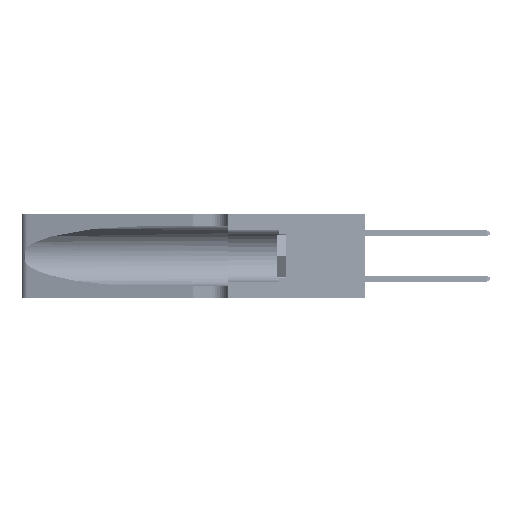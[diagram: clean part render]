
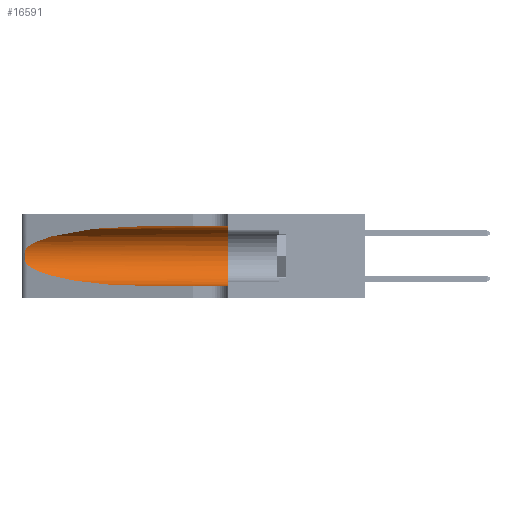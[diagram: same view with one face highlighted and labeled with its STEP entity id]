
A CAD part, left-side view. The second image highlights one B-rep face of the part: STEP entity #16591.
In plain terms, the highlighted cylindrical face has radius 3.308 mm (diameter 6.617 mm), a partial arc.
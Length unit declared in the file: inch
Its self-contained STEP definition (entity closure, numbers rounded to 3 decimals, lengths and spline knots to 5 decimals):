
#330 = VERTEX_POINT ( 'NONE', #38576 ) ;
#728 = EDGE_CURVE ( 'NONE', #48328, #16818, #50321, .T. ) ;
#2512 = CARTESIAN_POINT ( 'NONE',  ( 0.1305, 0.72297, 0.31525 ) ) ;
#3125 = DIRECTION ( 'NONE',  ( 0., 1., 0. ) ) ;
#3494 = CARTESIAN_POINT ( 'NONE',  ( 0.25854, 1.2359, 0.20912 ) ) ;
#3715 = VERTEX_POINT ( 'NONE', #28185 ) ;
#4630 = CARTESIAN_POINT ( 'NONE',  ( 0.1305, 0.72297, 0.05475 ) ) ;
#4679 = DIRECTION ( 'NONE',  ( 0., -1., 0. ) ) ;
#4864 = EDGE_CURVE ( 'NONE', #330, #8304, #37035, .T. ) ;
#4929 = DIRECTION ( 'NONE',  ( 0., -1., 0. ) ) ;
#5029 =( BOUNDED_CURVE ( )  B_SPLINE_CURVE ( 3, ( #16558, #36724, #28853, #4630 ),
 .UNSPECIFIED., .F., .F. ) 
 B_SPLINE_CURVE_WITH_KNOTS ( ( 4, 4 ),
 ( 3.44316, 4.71239 ),
 .UNSPECIFIED. ) 
 CURVE ( )  GEOMETRIC_REPRESENTATION_ITEM ( )  RATIONAL_B_SPLINE_CURVE ( ( 1., 0.87, 0.87, 1. ) ) 
 REPRESENTATION_ITEM ( '' )  );
#5839 = ORIENTED_EDGE ( 'NONE', *, *, #31354, .T. ) ;
#5960 = CARTESIAN_POINT ( 'NONE',  ( 0.1305, 0.35, 0.31525 ) ) ;
#7578 = CARTESIAN_POINT ( 'NONE',  ( 0.26075, 1.23896, 0.19203 ) ) ;
#8304 = VERTEX_POINT ( 'NONE', #19694 ) ;
#8867 = VECTOR ( 'NONE', #4679, 39.37008 ) ;
#8941 =( BOUNDED_CURVE ( )  B_SPLINE_CURVE ( 3, ( #2512, #34828, #46845, #22879 ),
 .UNSPECIFIED., .F., .T. ) 
 B_SPLINE_CURVE_WITH_KNOTS ( ( 4, 4 ),
 ( 1.5708, 2.84003 ),
 .UNSPECIFIED. ) 
 CURVE ( )  GEOMETRIC_REPRESENTATION_ITEM ( )  RATIONAL_B_SPLINE_CURVE ( ( 1., 0.87, 0.87, 1. ) ) 
 REPRESENTATION_ITEM ( '' )  );
#9006 = ORIENTED_EDGE ( 'NONE', *, *, #16191, .T. ) ;
#9106 = CARTESIAN_POINT ( 'NONE',  ( 0.1305, 1.61858, 0.05475 ) ) ;
#10333 = ORIENTED_EDGE ( 'NONE', *, *, #4864, .T. ) ;
#11710 = CARTESIAN_POINT ( 'NONE',  ( 0.26017, 1.23833, 0.17102 ) ) ;
#12333 = VERTEX_POINT ( 'NONE', #36916 ) ;
#14378 = VECTOR ( 'NONE', #41487, 39.37008 ) ;
#14620 = CIRCLE ( 'NONE', #47945, 0.13025 ) ;
#15626 = LINE ( 'NONE', #9106, #14378 ) ;
#15627 = CARTESIAN_POINT ( 'NONE',  ( 0.25487, 1.22718, 0.22369 ) ) ;
#15797 = CARTESIAN_POINT ( 'NONE',  ( 0.25789, 1.23486, 0.15765 ) ) ;
#15844 = CYLINDRICAL_SURFACE ( 'NONE', #50868, 0.13025 ) ;
#16191 = EDGE_CURVE ( 'NONE', #48328, #330, #8941, .T. ) ;
#16558 = CARTESIAN_POINT ( 'NONE',  ( 0.25487, 1.22718, 0.14631 ) ) ;
#16591 = ADVANCED_FACE ( 'NONE', ( #47780 ), #15844, .F. ) ;
#16697 = ORIENTED_EDGE ( 'NONE', *, *, #29116, .F. ) ;
#16818 = VERTEX_POINT ( 'NONE', #5960 ) ;
#17207 = CARTESIAN_POINT ( 'NONE',  ( 0.1305, 1.61858, 0.185 ) ) ;
#17241 = EDGE_LOOP ( 'NONE', ( #9006, #10333, #23610, #5839, #16697, #38031 ) ) ;
#19694 = CARTESIAN_POINT ( 'NONE',  ( 0.25487, 1.22718, 0.14631 ) ) ;
#19844 = CARTESIAN_POINT ( 'NONE',  ( 0.25555, 1.22993, 0.14849 ) ) ;
#22879 = CARTESIAN_POINT ( 'NONE',  ( 0.25487, 1.22718, 0.22369 ) ) ;
#23537 = CARTESIAN_POINT ( 'NONE',  ( 0.25555, 1.22994, 0.2215 ) ) ;
#23610 = ORIENTED_EDGE ( 'NONE', *, *, #38783, .T. ) ;
#24855 = CARTESIAN_POINT ( 'NONE',  ( 0.1305, 1.61858, 0.31525 ) ) ;
#27365 = CARTESIAN_POINT ( 'NONE',  ( 0.1305, 0.35, 0.185 ) ) ;
#27680 = CARTESIAN_POINT ( 'NONE',  ( 0.1305, 0.72297, 0.31525 ) ) ;
#27736 = CARTESIAN_POINT ( 'NONE',  ( 0.25787, 1.23484, 0.2124 ) ) ;
#28185 = CARTESIAN_POINT ( 'NONE',  ( 0.1305, 0.35, 0.05475 ) ) ;
#28853 = CARTESIAN_POINT ( 'NONE',  ( 0.18966, 0.96281, 0.05475 ) ) ;
#29116 = EDGE_CURVE ( 'NONE', #16818, #3715, #14620, .T. ) ;
#31354 = EDGE_CURVE ( 'NONE', #12333, #3715, #15626, .T. ) ;
#31406 = DIRECTION ( 'NONE',  ( 0., 0., 1. ) ) ;
#31770 = CARTESIAN_POINT ( 'NONE',  ( 0.26018, 1.23835, 0.19895 ) ) ;
#34828 = CARTESIAN_POINT ( 'NONE',  ( 0.18966, 0.96281, 0.31525 ) ) ;
#35795 = CARTESIAN_POINT ( 'NONE',  ( 0.26075, 1.23896, 0.178 ) ) ;
#36724 = CARTESIAN_POINT ( 'NONE',  ( 0.2373, 1.15595, 0.08982 ) ) ;
#36916 = CARTESIAN_POINT ( 'NONE',  ( 0.1305, 0.72297, 0.05475 ) ) ;
#37035 = B_SPLINE_CURVE_WITH_KNOTS ( 'NONE', 3,
 ( #15627, #23537, #51607, #27736, #3494, #31770, #7578, #35795, #11710, #39838, #15797, #43856, #19844, #47821 ),
 .UNSPECIFIED., .F., .F.,
 ( 4, 2, 2, 2, 2, 2, 4 ),
 ( 0., 0.00027, 0.00053, 0.00107, 0.0016, 0.00187, 0.00214 ),
 .UNSPECIFIED. ) ;
#37206 = DIRECTION ( 'NONE',  ( 0., 0., -1. ) ) ;
#38031 = ORIENTED_EDGE ( 'NONE', *, *, #728, .F. ) ;
#38576 = CARTESIAN_POINT ( 'NONE',  ( 0.25487, 1.22718, 0.22369 ) ) ;
#38783 = EDGE_CURVE ( 'NONE', #8304, #12333, #5029, .T. ) ;
#39838 = CARTESIAN_POINT ( 'NONE',  ( 0.25856, 1.23593, 0.16098 ) ) ;
#41487 = DIRECTION ( 'NONE',  ( 0., -1., 0. ) ) ;
#43856 = CARTESIAN_POINT ( 'NONE',  ( 0.25639, 1.23186, 0.15144 ) ) ;
#46845 = CARTESIAN_POINT ( 'NONE',  ( 0.2373, 1.15595, 0.28018 ) ) ;
#47780 = FACE_OUTER_BOUND ( 'NONE', #17241, .T. ) ;
#47821 = CARTESIAN_POINT ( 'NONE',  ( 0.25487, 1.22718, 0.14631 ) ) ;
#47945 = AXIS2_PLACEMENT_3D ( 'NONE', #27365, #3125, #31406 ) ;
#48328 = VERTEX_POINT ( 'NONE', #27680 ) ;
#50321 = LINE ( 'NONE', #24855, #8867 ) ;
#50868 = AXIS2_PLACEMENT_3D ( 'NONE', #17207, #4929, #37206 ) ;
#51607 = CARTESIAN_POINT ( 'NONE',  ( 0.25639, 1.23184, 0.21858 ) ) ;
